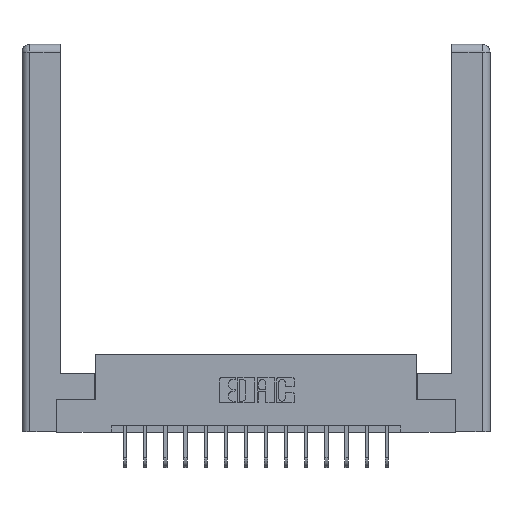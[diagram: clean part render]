
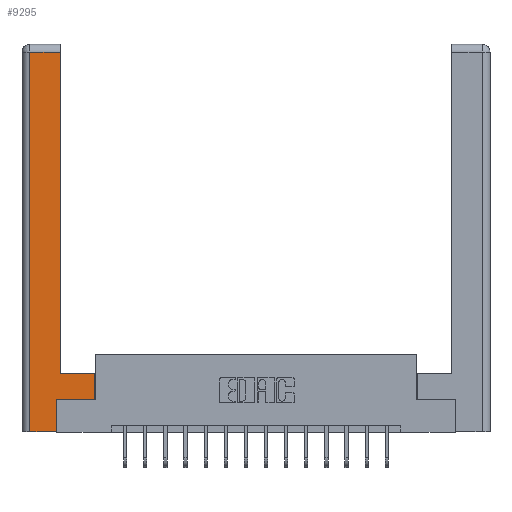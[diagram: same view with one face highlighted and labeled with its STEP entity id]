
A CAD part, top view. The second image highlights one B-rep face of the part: STEP entity #9295.
In plain terms, the highlighted planar face has unit normal (0, 0, 1).
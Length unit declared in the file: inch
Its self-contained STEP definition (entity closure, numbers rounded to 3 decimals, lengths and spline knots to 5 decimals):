
#66 = CARTESIAN_POINT ( 'NONE',  ( 0.565, 0.245, 0. ) ) ;
#727 = CARTESIAN_POINT ( 'NONE',  ( 0.565, 0.45, 0. ) ) ;
#784 = CARTESIAN_POINT ( 'NONE',  ( 0.0615, 2.94, 0. ) ) ;
#1010 = VERTEX_POINT ( 'NONE', #4730 ) ;
#1517 = VERTEX_POINT ( 'NONE', #727 ) ;
#1620 = CARTESIAN_POINT ( 'NONE',  ( 0.265, 0., 0. ) ) ;
#1714 = LINE ( 'NONE', #11216, #14673 ) ;
#1758 = DIRECTION ( 'NONE',  ( 0., -1., 0. ) ) ;
#1779 = ORIENTED_EDGE ( 'NONE', *, *, #10494, .T. ) ;
#1786 = VECTOR ( 'NONE', #1904, 39.37008 ) ;
#1904 = DIRECTION ( 'NONE',  ( 1., 0., 0. ) ) ;
#2249 = VERTEX_POINT ( 'NONE', #15190 ) ;
#2515 = VECTOR ( 'NONE', #12516, 39.37008 ) ;
#2535 = VECTOR ( 'NONE', #5630, 39.37008 ) ;
#2753 = EDGE_CURVE ( 'NONE', #15275, #1517, #1714, .T. ) ;
#2867 = ORIENTED_EDGE ( 'NONE', *, *, #8837, .T. ) ;
#2988 = LINE ( 'NONE', #8567, #1786 ) ;
#3458 = LINE ( 'NONE', #13184, #9687 ) ;
#3497 = LINE ( 'NONE', #11745, #8730 ) ;
#3545 = LINE ( 'NONE', #8204, #2535 ) ;
#3683 = PLANE ( 'NONE',  #10176 ) ;
#3882 = FACE_OUTER_BOUND ( 'NONE', #6290, .T. ) ;
#4204 = DIRECTION ( 'NONE',  ( 0., 1., 0. ) ) ;
#4206 = VERTEX_POINT ( 'NONE', #1620 ) ;
#4730 = CARTESIAN_POINT ( 'NONE',  ( 0.295, 0.45, 0. ) ) ;
#5407 = ORIENTED_EDGE ( 'NONE', *, *, #8668, .T. ) ;
#5413 = VERTEX_POINT ( 'NONE', #12498 ) ;
#5630 = DIRECTION ( 'NONE',  ( -1., 0., 0. ) ) ;
#5705 = VECTOR ( 'NONE', #11399, 39.37008 ) ;
#6131 = CARTESIAN_POINT ( 'NONE',  ( 0.0615, 2.94, 0. ) ) ;
#6280 = ORIENTED_EDGE ( 'NONE', *, *, #14407, .T. ) ;
#6290 = EDGE_LOOP ( 'NONE', ( #1779, #2867, #16331, #6628, #6587, #6280, #15988, #5407 ) ) ;
#6587 = ORIENTED_EDGE ( 'NONE', *, *, #7097, .T. ) ;
#6628 = ORIENTED_EDGE ( 'NONE', *, *, #10050, .T. ) ;
#6692 = VECTOR ( 'NONE', #8866, 39.37008 ) ;
#7097 = EDGE_CURVE ( 'NONE', #4206, #2249, #7174, .T. ) ;
#7174 = LINE ( 'NONE', #11678, #2515 ) ;
#7579 = VERTEX_POINT ( 'NONE', #784 ) ;
#8040 = EDGE_CURVE ( 'NONE', #7579, #13747, #3497, .T. ) ;
#8204 = CARTESIAN_POINT ( 'NONE',  ( 0.295, 0.45, 0. ) ) ;
#8272 = DIRECTION ( 'NONE',  ( 0., 0., -1. ) ) ;
#8343 = DIRECTION ( 'NONE',  ( -1., 0., 0. ) ) ;
#8567 = CARTESIAN_POINT ( 'NONE',  ( 0.565, 0.245, 0. ) ) ;
#8668 = EDGE_CURVE ( 'NONE', #1517, #1010, #3545, .T. ) ;
#8730 = VECTOR ( 'NONE', #1758, 39.37008 ) ;
#8837 = EDGE_CURVE ( 'NONE', #5413, #7579, #8929, .T. ) ;
#8866 = DIRECTION ( 'NONE',  ( 1., 0., 0. ) ) ;
#8929 = LINE ( 'NONE', #6131, #5705 ) ;
#9295 = ADVANCED_FACE ( 'NONE', ( #3882 ), #3683, .F. ) ;
#9687 = VECTOR ( 'NONE', #4204, 39.37008 ) ;
#9865 = DIRECTION ( 'NONE',  ( 0., 1., 0. ) ) ;
#10050 = EDGE_CURVE ( 'NONE', #13747, #4206, #11498, .T. ) ;
#10176 = AXIS2_PLACEMENT_3D ( 'NONE', #13376, #8272, #8343 ) ;
#10494 = EDGE_CURVE ( 'NONE', #1010, #5413, #3458, .T. ) ;
#11216 = CARTESIAN_POINT ( 'NONE',  ( 0.565, 0.45, 0. ) ) ;
#11330 = CARTESIAN_POINT ( 'NONE',  ( 0.265, 0., 0. ) ) ;
#11399 = DIRECTION ( 'NONE',  ( -1., 0., 0. ) ) ;
#11498 = LINE ( 'NONE', #11330, #6692 ) ;
#11678 = CARTESIAN_POINT ( 'NONE',  ( 0.265, 0.245, 0. ) ) ;
#11745 = CARTESIAN_POINT ( 'NONE',  ( 0.0615, 0., 0. ) ) ;
#12498 = CARTESIAN_POINT ( 'NONE',  ( 0.295, 2.94, 0. ) ) ;
#12516 = DIRECTION ( 'NONE',  ( 0., 1., 0. ) ) ;
#13184 = CARTESIAN_POINT ( 'NONE',  ( 0.295, 3., 0. ) ) ;
#13376 = CARTESIAN_POINT ( 'NONE',  ( 0., 0., 0. ) ) ;
#13747 = VERTEX_POINT ( 'NONE', #14927 ) ;
#14407 = EDGE_CURVE ( 'NONE', #2249, #15275, #2988, .T. ) ;
#14673 = VECTOR ( 'NONE', #9865, 39.37008 ) ;
#14927 = CARTESIAN_POINT ( 'NONE',  ( 0.0615, 0., 0. ) ) ;
#15190 = CARTESIAN_POINT ( 'NONE',  ( 0.265, 0.245, 0. ) ) ;
#15275 = VERTEX_POINT ( 'NONE', #66 ) ;
#15988 = ORIENTED_EDGE ( 'NONE', *, *, #2753, .T. ) ;
#16331 = ORIENTED_EDGE ( 'NONE', *, *, #8040, .T. ) ;
